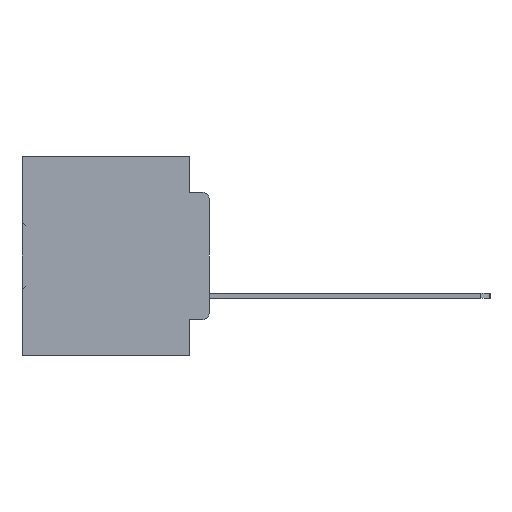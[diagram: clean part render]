
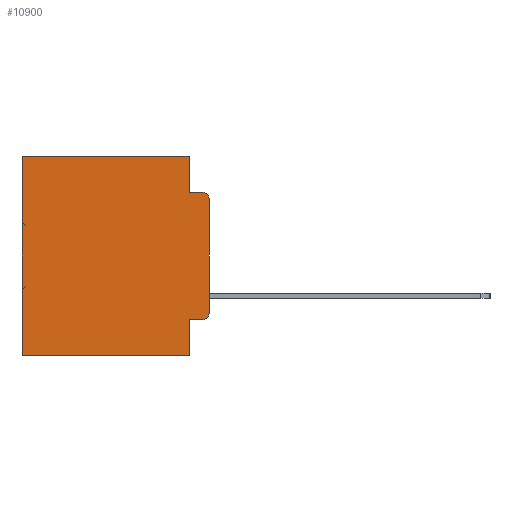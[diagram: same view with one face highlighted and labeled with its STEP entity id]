
A CAD part, left-side view. The second image highlights one B-rep face of the part: STEP entity #10900.
In plain terms, the highlighted planar face has unit normal (-1, 0, 0).
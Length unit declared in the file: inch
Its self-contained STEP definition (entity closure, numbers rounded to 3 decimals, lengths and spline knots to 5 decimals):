
#605 = CARTESIAN_POINT ( 'NONE',  ( 0.298, 0.02, -0.0885 ) ) ;
#685 = DIRECTION ( 'NONE',  ( 0., -1., 0. ) ) ;
#1481 = VERTEX_POINT ( 'NONE', #12282 ) ;
#1491 = EDGE_CURVE ( 'NONE', #31886, #7536, #14871, .T. ) ;
#2226 = CARTESIAN_POINT ( 'NONE',  ( 0.298, 0.02, -0.1085 ) ) ;
#2873 = CARTESIAN_POINT ( 'NONE',  ( 0.298, 0.051, 0. ) ) ;
#3185 = VECTOR ( 'NONE', #31719, 39.37008 ) ;
#3462 = DIRECTION ( 'NONE',  ( 0., 0., -1. ) ) ;
#4152 = CARTESIAN_POINT ( 'NONE',  ( 0.298, 0.02, -0.4115 ) ) ;
#4885 = DIRECTION ( 'NONE',  ( 0., 0., -1. ) ) ;
#5113 = DIRECTION ( 'NONE',  ( 0., 0., -1. ) ) ;
#5763 = ORIENTED_EDGE ( 'NONE', *, *, #26771, .F. ) ;
#5865 = CIRCLE ( 'NONE', #11515, 0.02 ) ;
#6275 = EDGE_CURVE ( 'NONE', #1481, #16980, #11442, .T. ) ;
#6328 = VERTEX_POINT ( 'NONE', #14917 ) ;
#6355 = VECTOR ( 'NONE', #685, 39.37008 ) ;
#7098 = LINE ( 'NONE', #35843, #13670 ) ;
#7234 = EDGE_CURVE ( 'NONE', #29408, #6328, #7865, .T. ) ;
#7314 = DIRECTION ( 'NONE',  ( 0., 0., -1. ) ) ;
#7536 = VERTEX_POINT ( 'NONE', #20192 ) ;
#7609 = ORIENTED_EDGE ( 'NONE', *, *, #33362, .T. ) ;
#7865 = LINE ( 'NONE', #24473, #29341 ) ;
#9015 = VERTEX_POINT ( 'NONE', #32791 ) ;
#9087 = CARTESIAN_POINT ( 'NONE',  ( 0.298, 0., 0. ) ) ;
#9364 = ORIENTED_EDGE ( 'NONE', *, *, #33351, .T. ) ;
#9391 = CARTESIAN_POINT ( 'NONE',  ( 0.298, 0., 0. ) ) ;
#10304 = DIRECTION ( 'NONE',  ( 0., 1., 0. ) ) ;
#10588 = ORIENTED_EDGE ( 'NONE', *, *, #7234, .T. ) ;
#10900 = ADVANCED_FACE ( 'NONE', ( #18028 ), #10949, .F. ) ;
#10949 = PLANE ( 'NONE',  #16058 ) ;
#11442 = LINE ( 'NONE', #9087, #18141 ) ;
#11515 = AXIS2_PLACEMENT_3D ( 'NONE', #14969, #34308, #17837 ) ;
#12282 = CARTESIAN_POINT ( 'NONE',  ( 0.298, 0., -0.1085 ) ) ;
#12922 = ORIENTED_EDGE ( 'NONE', *, *, #23055, .T. ) ;
#13670 = VECTOR ( 'NONE', #19606, 39.37008 ) ;
#13802 = CARTESIAN_POINT ( 'NONE',  ( 0.298, 0., 0. ) ) ;
#14028 = VECTOR ( 'NONE', #10304, 39.37008 ) ;
#14058 = EDGE_CURVE ( 'NONE', #17134, #24295, #28697, .T. ) ;
#14347 = CARTESIAN_POINT ( 'NONE',  ( 0.298, 0.051, -0.0885 ) ) ;
#14519 = LINE ( 'NONE', #14347, #28524 ) ;
#14857 = CARTESIAN_POINT ( 'NONE',  ( 0.298, 0.051, -0.4115 ) ) ;
#14871 = LINE ( 'NONE', #24007, #36008 ) ;
#14917 = CARTESIAN_POINT ( 'NONE',  ( 0.298, 0.473, -0.5 ) ) ;
#14969 = CARTESIAN_POINT ( 'NONE',  ( 0.298, 0.02, -0.3915 ) ) ;
#15920 = VERTEX_POINT ( 'NONE', #605 ) ;
#16058 = AXIS2_PLACEMENT_3D ( 'NONE', #13802, #35907, #19553 ) ;
#16897 = ORIENTED_EDGE ( 'NONE', *, *, #34959, .F. ) ;
#16980 = VERTEX_POINT ( 'NONE', #30509 ) ;
#17134 = VERTEX_POINT ( 'NONE', #25617 ) ;
#17837 = DIRECTION ( 'NONE',  ( 0., 0., -1. ) ) ;
#17892 = CIRCLE ( 'NONE', #19872, 0.02 ) ;
#18028 = FACE_OUTER_BOUND ( 'NONE', #20724, .T. ) ;
#18141 = VECTOR ( 'NONE', #3462, 39.37008 ) ;
#19553 = DIRECTION ( 'NONE',  ( 0., 0., -1. ) ) ;
#19606 = DIRECTION ( 'NONE',  ( 0., 0., -1. ) ) ;
#19872 = AXIS2_PLACEMENT_3D ( 'NONE', #2226, #22001, #5113 ) ;
#20192 = CARTESIAN_POINT ( 'NONE',  ( 0.298, 0.051, -0.0885 ) ) ;
#20404 = CARTESIAN_POINT ( 'NONE',  ( 0.298, 0.473, 0. ) ) ;
#20724 = EDGE_LOOP ( 'NONE', ( #27764, #12922, #5763, #21915, #7609, #10588, #29458, #16897, #32089, #9364 ) ) ;
#21915 = ORIENTED_EDGE ( 'NONE', *, *, #1491, .F. ) ;
#22001 = DIRECTION ( 'NONE',  ( -1., 0., 0. ) ) ;
#23055 = EDGE_CURVE ( 'NONE', #1481, #15920, #17892, .T. ) ;
#24007 = CARTESIAN_POINT ( 'NONE',  ( 0.298, 0.051, 0. ) ) ;
#24295 = VERTEX_POINT ( 'NONE', #4152 ) ;
#24473 = CARTESIAN_POINT ( 'NONE',  ( 0.298, 0.473, 0. ) ) ;
#25617 = CARTESIAN_POINT ( 'NONE',  ( 0.298, 0.051, -0.4115 ) ) ;
#26771 = EDGE_CURVE ( 'NONE', #7536, #15920, #14519, .T. ) ;
#27164 = CARTESIAN_POINT ( 'NONE',  ( 0.298, 0., -0.5 ) ) ;
#27764 = ORIENTED_EDGE ( 'NONE', *, *, #6275, .F. ) ;
#28524 = VECTOR ( 'NONE', #31017, 39.37008 ) ;
#28697 = LINE ( 'NONE', #14857, #6355 ) ;
#29341 = VECTOR ( 'NONE', #4885, 39.37008 ) ;
#29408 = VERTEX_POINT ( 'NONE', #20404 ) ;
#29458 = ORIENTED_EDGE ( 'NONE', *, *, #36029, .F. ) ;
#30509 = CARTESIAN_POINT ( 'NONE',  ( 0.298, 0., -0.3915 ) ) ;
#31017 = DIRECTION ( 'NONE',  ( 0., -1., 0. ) ) ;
#31719 = DIRECTION ( 'NONE',  ( 0., 1., 0. ) ) ;
#31886 = VERTEX_POINT ( 'NONE', #2873 ) ;
#32089 = ORIENTED_EDGE ( 'NONE', *, *, #14058, .T. ) ;
#32791 = CARTESIAN_POINT ( 'NONE',  ( 0.298, 0.051, -0.5 ) ) ;
#32862 = LINE ( 'NONE', #9391, #3185 ) ;
#33351 = EDGE_CURVE ( 'NONE', #24295, #16980, #5865, .T. ) ;
#33362 = EDGE_CURVE ( 'NONE', #31886, #29408, #32862, .T. ) ;
#34308 = DIRECTION ( 'NONE',  ( -1., 0., 0. ) ) ;
#34959 = EDGE_CURVE ( 'NONE', #17134, #9015, #7098, .T. ) ;
#35227 = LINE ( 'NONE', #27164, #14028 ) ;
#35843 = CARTESIAN_POINT ( 'NONE',  ( 0.298, 0.051, 0. ) ) ;
#35907 = DIRECTION ( 'NONE',  ( 1., 0., 0. ) ) ;
#36008 = VECTOR ( 'NONE', #7314, 39.37008 ) ;
#36029 = EDGE_CURVE ( 'NONE', #9015, #6328, #35227, .T. ) ;
